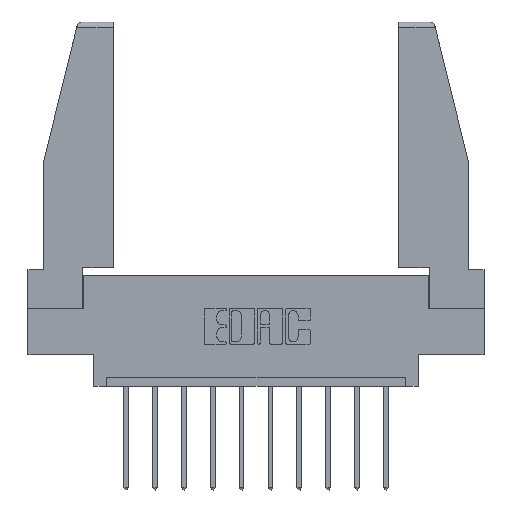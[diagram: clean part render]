
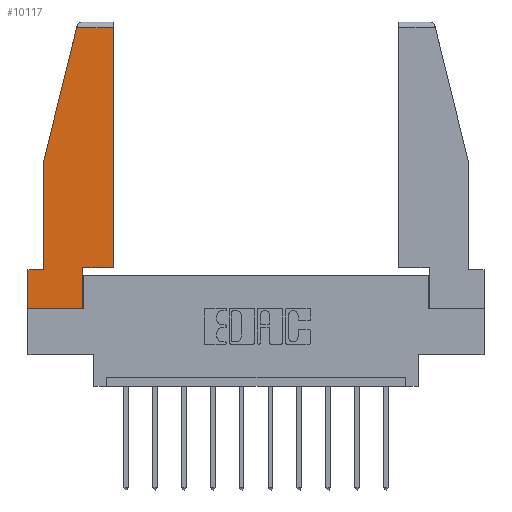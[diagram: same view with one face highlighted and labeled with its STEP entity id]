
A CAD part, top view. The second image highlights one B-rep face of the part: STEP entity #10117.
In plain terms, the highlighted planar face has unit normal (0, 0, 1).
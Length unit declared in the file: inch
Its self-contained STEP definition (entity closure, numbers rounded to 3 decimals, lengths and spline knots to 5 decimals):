
#2 = LINE ( 'NONE', #8782, #12088 ) ;
#254 = VECTOR ( 'NONE', #1862, 39.37008 ) ;
#268 = LINE ( 'NONE', #2600, #12720 ) ;
#279 = CARTESIAN_POINT ( 'NONE',  ( 0., 0., 0. ) ) ;
#395 = VERTEX_POINT ( 'NONE', #4884 ) ;
#481 = CARTESIAN_POINT ( 'NONE',  ( 0.297, 0., 0. ) ) ;
#562 = AXIS2_PLACEMENT_3D ( 'NONE', #6908, #12409, #12460 ) ;
#965 = ORIENTED_EDGE ( 'NONE', *, *, #8954, .T. ) ;
#1439 = LINE ( 'NONE', #8452, #254 ) ;
#1467 = VERTEX_POINT ( 'NONE', #5124 ) ;
#1494 = VERTEX_POINT ( 'NONE', #10435 ) ;
#1819 = VERTEX_POINT ( 'NONE', #9897 ) ;
#1862 = DIRECTION ( 'NONE',  ( 1., 0., 0. ) ) ;
#2330 = DIRECTION ( 'NONE',  ( -0.239, -0.971, 0. ) ) ;
#2344 = VERTEX_POINT ( 'NONE', #8865 ) ;
#2600 = CARTESIAN_POINT ( 'NONE',  ( 0.086, 0.8, 0. ) ) ;
#2608 = LINE ( 'NONE', #11530, #12690 ) ;
#2669 = DIRECTION ( 'NONE',  ( 0., 1., 0. ) ) ;
#2729 = CARTESIAN_POINT ( 'NONE',  ( 0.086, 0.8, 0. ) ) ;
#2836 = EDGE_CURVE ( 'NONE', #6621, #11001, #268, .T. ) ;
#2868 = CARTESIAN_POINT ( 'NONE',  ( 0.461, 0.223, 0. ) ) ;
#2887 = EDGE_CURVE ( 'NONE', #11001, #1819, #10991, .T. ) ;
#3195 = EDGE_CURVE ( 'NONE', #1494, #10845, #1439, .T. ) ;
#3211 = VECTOR ( 'NONE', #2669, 39.37008 ) ;
#4237 = EDGE_LOOP ( 'NONE', ( #965, #8803, #4663, #11124, #10787, #7732, #11372, #8786, #8731 ) ) ;
#4663 = ORIENTED_EDGE ( 'NONE', *, *, #5145, .T. ) ;
#4719 = VECTOR ( 'NONE', #11460, 39.37008 ) ;
#4724 = VECTOR ( 'NONE', #10653, 39.37008 ) ;
#4779 = LINE ( 'NONE', #279, #12949 ) ;
#4884 = CARTESIAN_POINT ( 'NONE',  ( 0., 0., 0. ) ) ;
#4938 = CARTESIAN_POINT ( 'NONE',  ( 0.086, 0.21, 0. ) ) ;
#5124 = CARTESIAN_POINT ( 'NONE',  ( 0.2636, 1.52, 0. ) ) ;
#5145 = EDGE_CURVE ( 'NONE', #1467, #6621, #2, .T. ) ;
#5224 = EDGE_CURVE ( 'NONE', #395, #2344, #4779, .T. ) ;
#5932 = DIRECTION ( 'NONE',  ( 0., -1., 0. ) ) ;
#6621 = VERTEX_POINT ( 'NONE', #2729 ) ;
#6669 = EDGE_CURVE ( 'NONE', #2344, #1494, #14191, .T. ) ;
#6858 = VERTEX_POINT ( 'NONE', #12372 ) ;
#6908 = CARTESIAN_POINT ( 'NONE',  ( 0., 0., 0. ) ) ;
#7048 = PLANE ( 'NONE',  #562 ) ;
#7357 = CARTESIAN_POINT ( 'NONE',  ( 0., 0.21, 0. ) ) ;
#7586 = EDGE_CURVE ( 'NONE', #6858, #1467, #10499, .T. ) ;
#7732 = ORIENTED_EDGE ( 'NONE', *, *, #13609, .T. ) ;
#7735 = VECTOR ( 'NONE', #5932, 39.37008 ) ;
#7924 = DIRECTION ( 'NONE',  ( 1., 0., 0. ) ) ;
#8186 = DIRECTION ( 'NONE',  ( 0., 1., 0. ) ) ;
#8452 = CARTESIAN_POINT ( 'NONE',  ( 0.297, 0.223, 0. ) ) ;
#8731 = ORIENTED_EDGE ( 'NONE', *, *, #3195, .T. ) ;
#8782 = CARTESIAN_POINT ( 'NONE',  ( 0.271, 1.55, 0. ) ) ;
#8786 = ORIENTED_EDGE ( 'NONE', *, *, #6669, .T. ) ;
#8803 = ORIENTED_EDGE ( 'NONE', *, *, #7586, .T. ) ;
#8865 = CARTESIAN_POINT ( 'NONE',  ( 0.297, 0., 0. ) ) ;
#8954 = EDGE_CURVE ( 'NONE', #10845, #6858, #2608, .T. ) ;
#9097 = CARTESIAN_POINT ( 'NONE',  ( 0., 0.21, 0. ) ) ;
#9690 = FACE_OUTER_BOUND ( 'NONE', #4237, .T. ) ;
#9897 = CARTESIAN_POINT ( 'NONE',  ( 0., 0.21, 0. ) ) ;
#10117 = ADVANCED_FACE ( 'NONE', ( #9690 ), #7048, .T. ) ;
#10435 = CARTESIAN_POINT ( 'NONE',  ( 0.297, 0.223, 0. ) ) ;
#10499 = LINE ( 'NONE', #10502, #4724 ) ;
#10502 = CARTESIAN_POINT ( 'NONE',  ( 0., 1.52, 0. ) ) ;
#10653 = DIRECTION ( 'NONE',  ( -1., 0., 0. ) ) ;
#10787 = ORIENTED_EDGE ( 'NONE', *, *, #2887, .T. ) ;
#10845 = VERTEX_POINT ( 'NONE', #2868 ) ;
#10991 = LINE ( 'NONE', #7357, #4719 ) ;
#11001 = VERTEX_POINT ( 'NONE', #4938 ) ;
#11124 = ORIENTED_EDGE ( 'NONE', *, *, #2836, .T. ) ;
#11314 = DIRECTION ( 'NONE',  ( 0., -1., 0. ) ) ;
#11372 = ORIENTED_EDGE ( 'NONE', *, *, #5224, .T. ) ;
#11460 = DIRECTION ( 'NONE',  ( -1., 0., 0. ) ) ;
#11530 = CARTESIAN_POINT ( 'NONE',  ( 0.461, 0.223, 0. ) ) ;
#12088 = VECTOR ( 'NONE', #2330, 39.37008 ) ;
#12305 = LINE ( 'NONE', #9097, #7735 ) ;
#12372 = CARTESIAN_POINT ( 'NONE',  ( 0.461, 1.52, 0. ) ) ;
#12409 = DIRECTION ( 'NONE',  ( 0., 0., 1. ) ) ;
#12460 = DIRECTION ( 'NONE',  ( 1., 0., 0. ) ) ;
#12690 = VECTOR ( 'NONE', #8186, 39.37008 ) ;
#12720 = VECTOR ( 'NONE', #11314, 39.37008 ) ;
#12949 = VECTOR ( 'NONE', #7924, 39.37008 ) ;
#13609 = EDGE_CURVE ( 'NONE', #1819, #395, #12305, .T. ) ;
#14191 = LINE ( 'NONE', #481, #3211 ) ;
